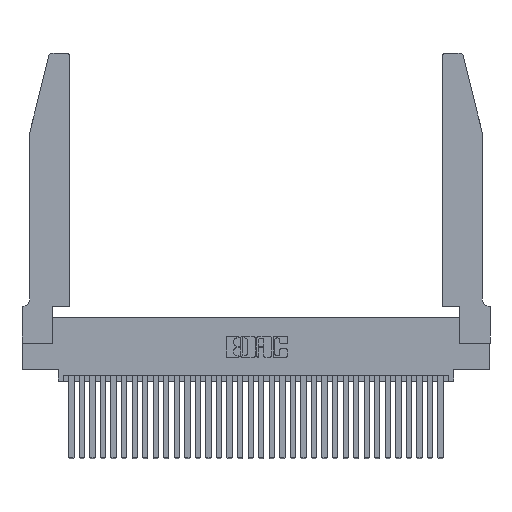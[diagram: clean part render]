
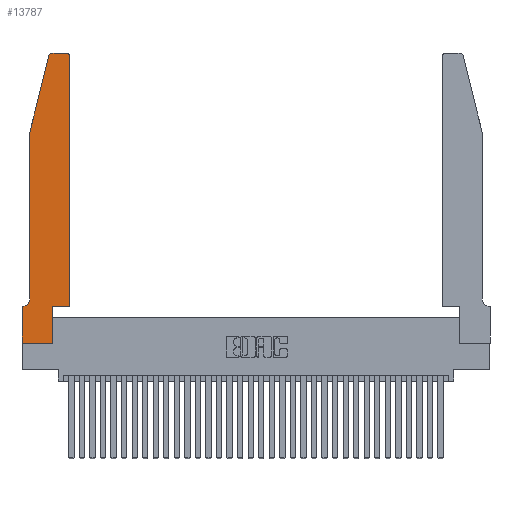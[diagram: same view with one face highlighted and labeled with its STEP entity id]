
A CAD part, top view. The second image highlights one B-rep face of the part: STEP entity #13787.
In plain terms, the highlighted planar face has unit normal (0, 0, 1).
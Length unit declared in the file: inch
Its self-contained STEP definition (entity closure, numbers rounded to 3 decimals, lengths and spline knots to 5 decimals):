
#250 = EDGE_CURVE ( 'NONE', #2480, #6279, #9228, .T. ) ;
#604 = CARTESIAN_POINT ( 'NONE',  ( 0.2605, 2.75, 0.37 ) ) ;
#863 = CARTESIAN_POINT ( 'NONE',  ( 0.0755, 2., 0.37 ) ) ;
#1309 = EDGE_CURVE ( 'NONE', #6279, #13562, #32950, .T. ) ;
#1423 = VERTEX_POINT ( 'NONE', #14629 ) ;
#1845 = DIRECTION ( 'NONE',  ( -1., 0., 0. ) ) ;
#2297 = CARTESIAN_POINT ( 'NONE',  ( 0.4505, 0.35, 0.37 ) ) ;
#2480 = VERTEX_POINT ( 'NONE', #18200 ) ;
#2554 = DIRECTION ( 'NONE',  ( 0., 0., 1. ) ) ;
#2947 = EDGE_CURVE ( 'NONE', #21210, #20397, #23642, .T. ) ;
#3069 = ORIENTED_EDGE ( 'NONE', *, *, #17058, .T. ) ;
#3322 = VECTOR ( 'NONE', #14288, 39.37008 ) ;
#3792 = AXIS2_PLACEMENT_3D ( 'NONE', #25718, #4559, #21451 ) ;
#3852 = ORIENTED_EDGE ( 'NONE', *, *, #31473, .T. ) ;
#4292 = CARTESIAN_POINT ( 'NONE',  ( 0., 0.35, 0.37 ) ) ;
#4541 = ORIENTED_EDGE ( 'NONE', *, *, #32316, .T. ) ;
#4559 = DIRECTION ( 'NONE',  ( 0., 0., 1. ) ) ;
#4777 = VECTOR ( 'NONE', #8306, 39.37008 ) ;
#4824 = ORIENTED_EDGE ( 'NONE', *, *, #25296, .T. ) ;
#4858 = ORIENTED_EDGE ( 'NONE', *, *, #18499, .T. ) ;
#5227 = ORIENTED_EDGE ( 'NONE', *, *, #21709, .T. ) ;
#5833 = LINE ( 'NONE', #26709, #18906 ) ;
#5999 = LINE ( 'NONE', #15520, #20659 ) ;
#6279 = VERTEX_POINT ( 'NONE', #15182 ) ;
#6509 = EDGE_LOOP ( 'NONE', ( #4541, #3852, #5227, #3069, #4824, #26426, #22776, #24425, #16340, #4858, #13544, #9925 ) ) ;
#7114 = VERTEX_POINT ( 'NONE', #8205 ) ;
#7282 = FACE_OUTER_BOUND ( 'NONE', #6509, .T. ) ;
#8169 = AXIS2_PLACEMENT_3D ( 'NONE', #14615, #32571, #17177 ) ;
#8205 = CARTESIAN_POINT ( 'NONE',  ( 0.2865, 0.35, 0.37 ) ) ;
#8306 = DIRECTION ( 'NONE',  ( 0., 1., 0. ) ) ;
#8539 = DIRECTION ( 'NONE',  ( 0., 0., 1. ) ) ;
#9228 = LINE ( 'NONE', #2297, #22114 ) ;
#9246 = LINE ( 'NONE', #13104, #29022 ) ;
#9608 = EDGE_CURVE ( 'NONE', #20397, #25432, #5833, .T. ) ;
#9925 = ORIENTED_EDGE ( 'NONE', *, *, #1309, .T. ) ;
#11094 = CARTESIAN_POINT ( 'NONE',  ( 0.0755, 2., 0.37 ) ) ;
#11558 = CARTESIAN_POINT ( 'NONE',  ( 0.0755, 2., 0.37 ) ) ;
#13104 = CARTESIAN_POINT ( 'NONE',  ( 0.4505, 0.35, 0.37 ) ) ;
#13544 = ORIENTED_EDGE ( 'NONE', *, *, #250, .T. ) ;
#13552 = VECTOR ( 'NONE', #1845, 39.37008 ) ;
#13562 = VERTEX_POINT ( 'NONE', #20027 ) ;
#13787 = ADVANCED_FACE ( 'NONE', ( #7282 ), #31147, .T. ) ;
#14288 = DIRECTION ( 'NONE',  ( 0., -1., 0. ) ) ;
#14615 = CARTESIAN_POINT ( 'NONE',  ( 0.0055, 0.42, 0.37 ) ) ;
#14629 = CARTESIAN_POINT ( 'NONE',  ( 0.2865, 0., 0.37 ) ) ;
#14815 = CARTESIAN_POINT ( 'NONE',  ( 0.284, 2.75, 0.37 ) ) ;
#15182 = CARTESIAN_POINT ( 'NONE',  ( 0.4505, 2.72, 0.37 ) ) ;
#15520 = CARTESIAN_POINT ( 'NONE',  ( 0., 0., 0.37 ) ) ;
#15687 = DIRECTION ( 'NONE',  ( 1., 0., 0. ) ) ;
#15939 = DIRECTION ( 'NONE',  ( 0., 1., 0. ) ) ;
#16340 = ORIENTED_EDGE ( 'NONE', *, *, #31423, .T. ) ;
#16435 = CARTESIAN_POINT ( 'NONE',  ( 0.0055, 0.35, 0.37 ) ) ;
#17058 = EDGE_CURVE ( 'NONE', #23314, #20623, #25869, .T. ) ;
#17177 = DIRECTION ( 'NONE',  ( -1., 0., 0. ) ) ;
#18086 = DIRECTION ( 'NONE',  ( 1., 0., 0. ) ) ;
#18200 = CARTESIAN_POINT ( 'NONE',  ( 0.4505, 0.35, 0.37 ) ) ;
#18321 = CARTESIAN_POINT ( 'NONE',  ( 0., 0.35, 0.37 ) ) ;
#18499 = EDGE_CURVE ( 'NONE', #7114, #2480, #9246, .T. ) ;
#18885 = CARTESIAN_POINT ( 'NONE',  ( 0.25487, 2.72718, 0.37 ) ) ;
#18906 = VECTOR ( 'NONE', #29291, 39.37008 ) ;
#19087 = DIRECTION ( 'NONE',  ( -1., 0., 0. ) ) ;
#19973 = LINE ( 'NONE', #11094, #26065 ) ;
#20027 = CARTESIAN_POINT ( 'NONE',  ( 0.4205, 2.75, 0.37 ) ) ;
#20397 = VERTEX_POINT ( 'NONE', #4292 ) ;
#20623 = VERTEX_POINT ( 'NONE', #28670 ) ;
#20659 = VECTOR ( 'NONE', #18086, 39.37008 ) ;
#20895 = DIRECTION ( 'NONE',  ( 1., 0., 0. ) ) ;
#21210 = VERTEX_POINT ( 'NONE', #16435 ) ;
#21440 = DIRECTION ( 'NONE',  ( -0.239, -0.971, 0. ) ) ;
#21451 = DIRECTION ( 'NONE',  ( 1., 0., 0. ) ) ;
#21709 = EDGE_CURVE ( 'NONE', #25129, #23314, #19973, .T. ) ;
#22114 = VECTOR ( 'NONE', #15939, 39.37008 ) ;
#22776 = ORIENTED_EDGE ( 'NONE', *, *, #9608, .T. ) ;
#22952 = CIRCLE ( 'NONE', #8169, 0.07 ) ;
#23132 = CIRCLE ( 'NONE', #26687, 0.03 ) ;
#23314 = VERTEX_POINT ( 'NONE', #11558 ) ;
#23642 = LINE ( 'NONE', #27939, #13552 ) ;
#23789 = CARTESIAN_POINT ( 'NONE',  ( 0.2865, 0.35, 0.37 ) ) ;
#24012 = CARTESIAN_POINT ( 'NONE',  ( 0.284, 2.72, 0.37 ) ) ;
#24425 = ORIENTED_EDGE ( 'NONE', *, *, #32066, .T. ) ;
#24714 = VECTOR ( 'NONE', #19087, 39.37008 ) ;
#25129 = VERTEX_POINT ( 'NONE', #18885 ) ;
#25207 = CARTESIAN_POINT ( 'NONE',  ( 0., 0., 0.37 ) ) ;
#25296 = EDGE_CURVE ( 'NONE', #20623, #21210, #22952, .T. ) ;
#25432 = VERTEX_POINT ( 'NONE', #25207 ) ;
#25718 = CARTESIAN_POINT ( 'NONE',  ( 0.4205, 2.72, 0.37 ) ) ;
#25869 = LINE ( 'NONE', #863, #3322 ) ;
#26065 = VECTOR ( 'NONE', #21440, 39.37008 ) ;
#26426 = ORIENTED_EDGE ( 'NONE', *, *, #2947, .T. ) ;
#26619 = DIRECTION ( 'NONE',  ( 1., 0., 0. ) ) ;
#26687 = AXIS2_PLACEMENT_3D ( 'NONE', #24012, #8539, #26619 ) ;
#26709 = CARTESIAN_POINT ( 'NONE',  ( 0., 0., 0.37 ) ) ;
#27939 = CARTESIAN_POINT ( 'NONE',  ( 0.0755, 0.35, 0.37 ) ) ;
#28670 = CARTESIAN_POINT ( 'NONE',  ( 0.0755, 0.42, 0.37 ) ) ;
#29022 = VECTOR ( 'NONE', #15687, 39.37008 ) ;
#29291 = DIRECTION ( 'NONE',  ( 0., -1., 0. ) ) ;
#29995 = LINE ( 'NONE', #23789, #4777 ) ;
#30711 = LINE ( 'NONE', #604, #24714 ) ;
#31095 = VERTEX_POINT ( 'NONE', #14815 ) ;
#31147 = PLANE ( 'NONE',  #33458 ) ;
#31423 = EDGE_CURVE ( 'NONE', #1423, #7114, #29995, .T. ) ;
#31473 = EDGE_CURVE ( 'NONE', #31095, #25129, #23132, .T. ) ;
#32066 = EDGE_CURVE ( 'NONE', #25432, #1423, #5999, .T. ) ;
#32316 = EDGE_CURVE ( 'NONE', #13562, #31095, #30711, .T. ) ;
#32571 = DIRECTION ( 'NONE',  ( 0., 0., -1. ) ) ;
#32950 = CIRCLE ( 'NONE', #3792, 0.03 ) ;
#33458 = AXIS2_PLACEMENT_3D ( 'NONE', #18321, #2554, #20895 ) ;
